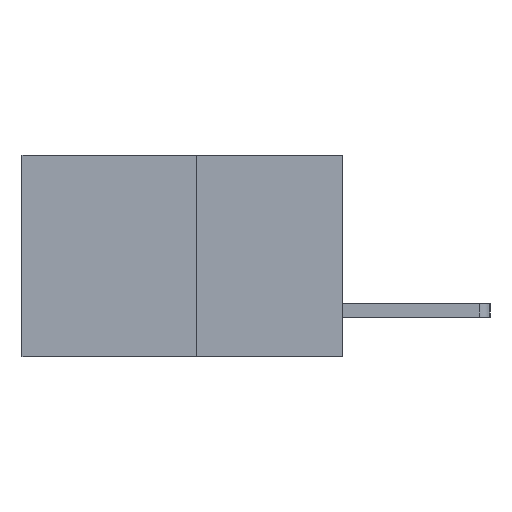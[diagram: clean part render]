
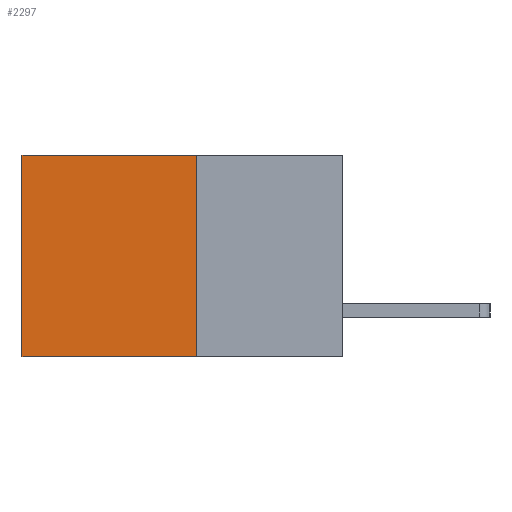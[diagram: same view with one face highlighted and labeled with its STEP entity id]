
A CAD part, left-side view. The second image highlights one B-rep face of the part: STEP entity #2297.
In plain terms, the highlighted planar face has unit normal (-1, 0, 0).
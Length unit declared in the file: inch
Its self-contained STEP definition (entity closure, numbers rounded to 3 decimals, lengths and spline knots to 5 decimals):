
#261 = ORIENTED_EDGE ( 'NONE', *, *, #4745, .F. ) ;
#637 = EDGE_CURVE ( 'NONE', #11841, #1555, #8309, .T. ) ;
#971 = AXIS2_PLACEMENT_3D ( 'NONE', #9415, #9483, #9251 ) ;
#1275 = CARTESIAN_POINT ( 'NONE',  ( 0.277, 0.27, -0.37 ) ) ;
#1555 = VERTEX_POINT ( 'NONE', #9471 ) ;
#1567 = VECTOR ( 'NONE', #3543, 39.37008 ) ;
#2297 = ADVANCED_FACE ( 'NONE', ( #10763 ), #9357, .F. ) ;
#3170 = VECTOR ( 'NONE', #4312, 39.37008 ) ;
#3328 = CARTESIAN_POINT ( 'NONE',  ( 0.277, 0.59, -0.37 ) ) ;
#3543 = DIRECTION ( 'NONE',  ( 0., 0., -1. ) ) ;
#3611 = CARTESIAN_POINT ( 'NONE',  ( 0.277, 0.59, -0.37 ) ) ;
#4312 = DIRECTION ( 'NONE',  ( 0., 1., 0. ) ) ;
#4616 = DIRECTION ( 'NONE',  ( 0., 1., 0. ) ) ;
#4745 = EDGE_CURVE ( 'NONE', #1555, #5389, #10407, .T. ) ;
#5272 = VERTEX_POINT ( 'NONE', #8646 ) ;
#5307 = EDGE_CURVE ( 'NONE', #11841, #5272, #7388, .T. ) ;
#5389 = VERTEX_POINT ( 'NONE', #3328 ) ;
#5688 = DIRECTION ( 'NONE',  ( 0., 0., -1. ) ) ;
#5954 = CARTESIAN_POINT ( 'NONE',  ( 0.277, 0.27, -0.37 ) ) ;
#7060 = EDGE_CURVE ( 'NONE', #5272, #5389, #11596, .T. ) ;
#7388 = LINE ( 'NONE', #10320, #9180 ) ;
#7901 = ORIENTED_EDGE ( 'NONE', *, *, #637, .F. ) ;
#8309 = LINE ( 'NONE', #1275, #11972 ) ;
#8646 = CARTESIAN_POINT ( 'NONE',  ( 0.277, 0.59, 0. ) ) ;
#9180 = VECTOR ( 'NONE', #4616, 39.37008 ) ;
#9251 = DIRECTION ( 'NONE',  ( 0., 0., -1. ) ) ;
#9357 = PLANE ( 'NONE',  #971 ) ;
#9415 = CARTESIAN_POINT ( 'NONE',  ( 0.277, 0.27, -0.37 ) ) ;
#9471 = CARTESIAN_POINT ( 'NONE',  ( 0.277, 0.27, -0.37 ) ) ;
#9483 = DIRECTION ( 'NONE',  ( 1., 0., 0. ) ) ;
#9981 = ORIENTED_EDGE ( 'NONE', *, *, #7060, .T. ) ;
#10248 = ORIENTED_EDGE ( 'NONE', *, *, #5307, .T. ) ;
#10320 = CARTESIAN_POINT ( 'NONE',  ( 0.277, 0.27, 0. ) ) ;
#10407 = LINE ( 'NONE', #5954, #3170 ) ;
#10763 = FACE_OUTER_BOUND ( 'NONE', #11373, .T. ) ;
#11023 = CARTESIAN_POINT ( 'NONE',  ( 0.277, 0.27, 0. ) ) ;
#11373 = EDGE_LOOP ( 'NONE', ( #9981, #261, #7901, #10248 ) ) ;
#11596 = LINE ( 'NONE', #3611, #1567 ) ;
#11841 = VERTEX_POINT ( 'NONE', #11023 ) ;
#11972 = VECTOR ( 'NONE', #5688, 39.37008 ) ;
